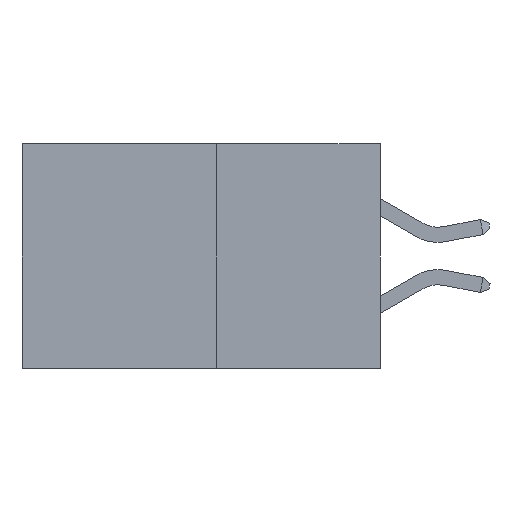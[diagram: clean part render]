
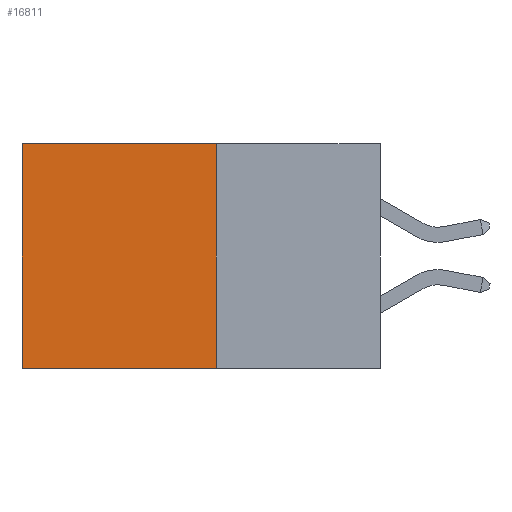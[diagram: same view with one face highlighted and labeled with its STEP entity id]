
A CAD part, left-side view. The second image highlights one B-rep face of the part: STEP entity #16811.
In plain terms, the highlighted planar face has unit normal (-1, 0, 0).
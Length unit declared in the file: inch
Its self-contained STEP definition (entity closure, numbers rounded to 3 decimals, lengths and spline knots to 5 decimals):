
#1198 = LINE ( 'NONE', #7670, #19282 ) ;
#2099 = CARTESIAN_POINT ( 'NONE',  ( 0.277, 0.27, -0.37 ) ) ;
#3374 = CARTESIAN_POINT ( 'NONE',  ( 0.277, 0.27, -0.37 ) ) ;
#3616 = CARTESIAN_POINT ( 'NONE',  ( 0.277, 0.59, 0. ) ) ;
#3672 = CARTESIAN_POINT ( 'NONE',  ( 0.277, 0.59, -0.37 ) ) ;
#4152 = CARTESIAN_POINT ( 'NONE',  ( 0.277, 0.27, 0. ) ) ;
#4238 = DIRECTION ( 'NONE',  ( 1., 0., 0. ) ) ;
#4543 = VERTEX_POINT ( 'NONE', #3616 ) ;
#4593 = ORIENTED_EDGE ( 'NONE', *, *, #13689, .F. ) ;
#4779 = DIRECTION ( 'NONE',  ( 0., 1., 0. ) ) ;
#5328 = EDGE_CURVE ( 'NONE', #15983, #4543, #29688, .T. ) ;
#5787 = CARTESIAN_POINT ( 'NONE',  ( 0.277, 0.59, -0.37 ) ) ;
#6081 = DIRECTION ( 'NONE',  ( 0., 0., -1. ) ) ;
#6134 = EDGE_LOOP ( 'NONE', ( #13962, #18425, #4593, #24309 ) ) ;
#7670 = CARTESIAN_POINT ( 'NONE',  ( 0.277, 0.27, -0.37 ) ) ;
#8204 = VERTEX_POINT ( 'NONE', #5787 ) ;
#10058 = DIRECTION ( 'NONE',  ( 0., 0., -1. ) ) ;
#13041 = AXIS2_PLACEMENT_3D ( 'NONE', #22901, #4238, #20674 ) ;
#13689 = EDGE_CURVE ( 'NONE', #15983, #26571, #1198, .T. ) ;
#13962 = ORIENTED_EDGE ( 'NONE', *, *, #25874, .T. ) ;
#15861 = CARTESIAN_POINT ( 'NONE',  ( 0.277, 0.27, 0. ) ) ;
#15884 = FACE_OUTER_BOUND ( 'NONE', #6134, .T. ) ;
#15983 = VERTEX_POINT ( 'NONE', #15861 ) ;
#16811 = ADVANCED_FACE ( 'NONE', ( #15884 ), #25229, .F. ) ;
#18425 = ORIENTED_EDGE ( 'NONE', *, *, #26207, .F. ) ;
#19282 = VECTOR ( 'NONE', #10058, 39.37008 ) ;
#20674 = DIRECTION ( 'NONE',  ( 0., 0., -1. ) ) ;
#22901 = CARTESIAN_POINT ( 'NONE',  ( 0.277, 0.27, -0.37 ) ) ;
#23383 = VECTOR ( 'NONE', #25526, 39.37008 ) ;
#24309 = ORIENTED_EDGE ( 'NONE', *, *, #5328, .T. ) ;
#25229 = PLANE ( 'NONE',  #13041 ) ;
#25526 = DIRECTION ( 'NONE',  ( 0., 1., 0. ) ) ;
#25874 = EDGE_CURVE ( 'NONE', #4543, #8204, #26668, .T. ) ;
#26207 = EDGE_CURVE ( 'NONE', #26571, #8204, #30266, .T. ) ;
#26571 = VERTEX_POINT ( 'NONE', #3374 ) ;
#26668 = LINE ( 'NONE', #3672, #27382 ) ;
#27382 = VECTOR ( 'NONE', #6081, 39.37008 ) ;
#28974 = VECTOR ( 'NONE', #4779, 39.37008 ) ;
#29688 = LINE ( 'NONE', #4152, #28974 ) ;
#30266 = LINE ( 'NONE', #2099, #23383 ) ;
